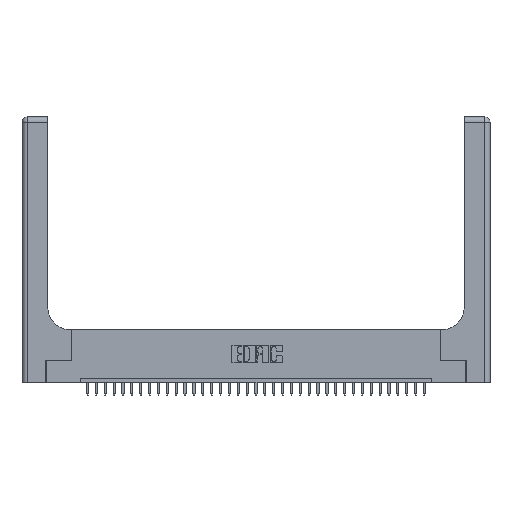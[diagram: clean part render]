
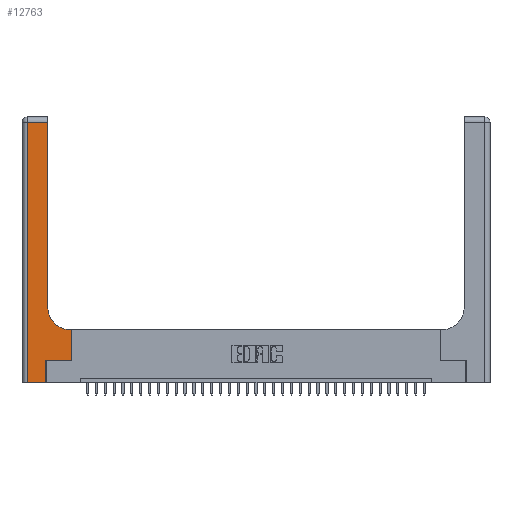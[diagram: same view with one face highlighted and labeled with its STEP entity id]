
A CAD part, top view. The second image highlights one B-rep face of the part: STEP entity #12763.
In plain terms, the highlighted planar face has unit normal (0, 0, 1).
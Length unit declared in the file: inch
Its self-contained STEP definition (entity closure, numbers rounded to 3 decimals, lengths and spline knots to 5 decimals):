
#510 = ORIENTED_EDGE ( 'NONE', *, *, #26098, .T. ) ;
#690 = DIRECTION ( 'NONE',  ( 0., -1., 0. ) ) ;
#904 = DIRECTION ( 'NONE',  ( 0., 1., 0. ) ) ;
#953 = CARTESIAN_POINT ( 'NONE',  ( 0.06, 2.94, 0.37 ) ) ;
#1590 = VECTOR ( 'NONE', #904, 39.37008 ) ;
#1672 = VECTOR ( 'NONE', #20255, 39.37008 ) ;
#1898 = VERTEX_POINT ( 'NONE', #5432 ) ;
#2061 = CARTESIAN_POINT ( 'NONE',  ( 0.5585, 0.25, 0.37 ) ) ;
#2205 = VERTEX_POINT ( 'NONE', #29512 ) ;
#3306 = DIRECTION ( 'NONE',  ( -1., 0., 0. ) ) ;
#4674 = VERTEX_POINT ( 'NONE', #17104 ) ;
#4925 = EDGE_CURVE ( 'NONE', #16381, #30464, #13049, .T. ) ;
#5249 = ORIENTED_EDGE ( 'NONE', *, *, #15325, .T. ) ;
#5289 = EDGE_CURVE ( 'NONE', #33606, #16381, #10520, .T. ) ;
#5432 = CARTESIAN_POINT ( 'NONE',  ( 0.2915, 2.94, 0.37 ) ) ;
#5795 = VECTOR ( 'NONE', #20499, 39.37008 ) ;
#5880 = ORIENTED_EDGE ( 'NONE', *, *, #18802, .T. ) ;
#6385 = ORIENTED_EDGE ( 'NONE', *, *, #15056, .T. ) ;
#6497 = VECTOR ( 'NONE', #15340, 39.37008 ) ;
#8043 = VECTOR ( 'NONE', #11106, 39.37008 ) ;
#8737 = CARTESIAN_POINT ( 'NONE',  ( 0.269, 0.25, 0.37 ) ) ;
#8873 = ORIENTED_EDGE ( 'NONE', *, *, #25899, .T. ) ;
#10072 = AXIS2_PLACEMENT_3D ( 'NONE', #18997, #19107, #11286 ) ;
#10520 = LINE ( 'NONE', #14643, #1590 ) ;
#10595 = LINE ( 'NONE', #8737, #34169 ) ;
#11106 = DIRECTION ( 'NONE',  ( -1., 0., 0. ) ) ;
#11286 = DIRECTION ( 'NONE',  ( 1., 0., 0. ) ) ;
#12527 = CARTESIAN_POINT ( 'NONE',  ( 0.269, 0., 0.37 ) ) ;
#12763 = ADVANCED_FACE ( 'NONE', ( #23795 ), #27819, .F. ) ;
#12805 = ORIENTED_EDGE ( 'NONE', *, *, #21710, .T. ) ;
#13049 = LINE ( 'NONE', #19148, #5795 ) ;
#13137 = CARTESIAN_POINT ( 'NONE',  ( 0.5585, 0.6, 0.37 ) ) ;
#13842 = CARTESIAN_POINT ( 'NONE',  ( 0.06, 3., 0.37 ) ) ;
#14229 = CARTESIAN_POINT ( 'NONE',  ( 0., 3., 0.37 ) ) ;
#14412 = DIRECTION ( 'NONE',  ( 1., 0., 0. ) ) ;
#14643 = CARTESIAN_POINT ( 'NONE',  ( 0.5585, 0.25, 0.37 ) ) ;
#15056 = EDGE_CURVE ( 'NONE', #1898, #24829, #15195, .T. ) ;
#15195 = LINE ( 'NONE', #31955, #8043 ) ;
#15325 = EDGE_CURVE ( 'NONE', #2205, #33606, #10595, .T. ) ;
#15340 = DIRECTION ( 'NONE',  ( 0., 1., 0. ) ) ;
#16381 = VERTEX_POINT ( 'NONE', #13137 ) ;
#17104 = CARTESIAN_POINT ( 'NONE',  ( 0.2915, 0.85, 0.37 ) ) ;
#18511 = VECTOR ( 'NONE', #690, 39.37008 ) ;
#18802 = EDGE_CURVE ( 'NONE', #4674, #1898, #19522, .T. ) ;
#18900 = CIRCLE ( 'NONE', #10072, 0.25 ) ;
#18997 = CARTESIAN_POINT ( 'NONE',  ( 0.5415, 0.85, 0.37 ) ) ;
#19107 = DIRECTION ( 'NONE',  ( 0., 0., -1. ) ) ;
#19148 = CARTESIAN_POINT ( 'NONE',  ( 0.2915, 0.6, 0.37 ) ) ;
#19522 = LINE ( 'NONE', #31102, #6497 ) ;
#20255 = DIRECTION ( 'NONE',  ( 0., 1., 0. ) ) ;
#20499 = DIRECTION ( 'NONE',  ( -1., 0., 0. ) ) ;
#20935 = ORIENTED_EDGE ( 'NONE', *, *, #5289, .T. ) ;
#21710 = EDGE_CURVE ( 'NONE', #25315, #2205, #23173, .T. ) ;
#22215 = EDGE_CURVE ( 'NONE', #30464, #4674, #18900, .T. ) ;
#22314 = VERTEX_POINT ( 'NONE', #31119 ) ;
#23173 = LINE ( 'NONE', #12527, #1672 ) ;
#23639 = EDGE_LOOP ( 'NONE', ( #5880, #6385, #8873, #510, #12805, #5249, #20935, #30538, #30818 ) ) ;
#23795 = FACE_OUTER_BOUND ( 'NONE', #23639, .T. ) ;
#24185 = CARTESIAN_POINT ( 'NONE',  ( 0.5415, 0.6, 0.37 ) ) ;
#24829 = VERTEX_POINT ( 'NONE', #953 ) ;
#25315 = VERTEX_POINT ( 'NONE', #29871 ) ;
#25658 = LINE ( 'NONE', #13842, #18511 ) ;
#25899 = EDGE_CURVE ( 'NONE', #24829, #22314, #25658, .T. ) ;
#25926 = CARTESIAN_POINT ( 'NONE',  ( 0., 0., 0.37 ) ) ;
#26079 = LINE ( 'NONE', #25926, #28169 ) ;
#26098 = EDGE_CURVE ( 'NONE', #22314, #25315, #26079, .T. ) ;
#27819 = PLANE ( 'NONE',  #28157 ) ;
#28157 = AXIS2_PLACEMENT_3D ( 'NONE', #14229, #33293, #3306 ) ;
#28169 = VECTOR ( 'NONE', #28282, 39.37008 ) ;
#28282 = DIRECTION ( 'NONE',  ( 1., 0., 0. ) ) ;
#29512 = CARTESIAN_POINT ( 'NONE',  ( 0.269, 0.25, 0.37 ) ) ;
#29871 = CARTESIAN_POINT ( 'NONE',  ( 0.269, 0., 0.37 ) ) ;
#30464 = VERTEX_POINT ( 'NONE', #24185 ) ;
#30538 = ORIENTED_EDGE ( 'NONE', *, *, #4925, .T. ) ;
#30818 = ORIENTED_EDGE ( 'NONE', *, *, #22215, .T. ) ;
#31102 = CARTESIAN_POINT ( 'NONE',  ( 0.2915, 3., 0.37 ) ) ;
#31119 = CARTESIAN_POINT ( 'NONE',  ( 0.06, 0., 0.37 ) ) ;
#31955 = CARTESIAN_POINT ( 'NONE',  ( 0., 2.94, 0.37 ) ) ;
#33293 = DIRECTION ( 'NONE',  ( 0., 0., -1. ) ) ;
#33606 = VERTEX_POINT ( 'NONE', #2061 ) ;
#34169 = VECTOR ( 'NONE', #14412, 39.37008 ) ;
